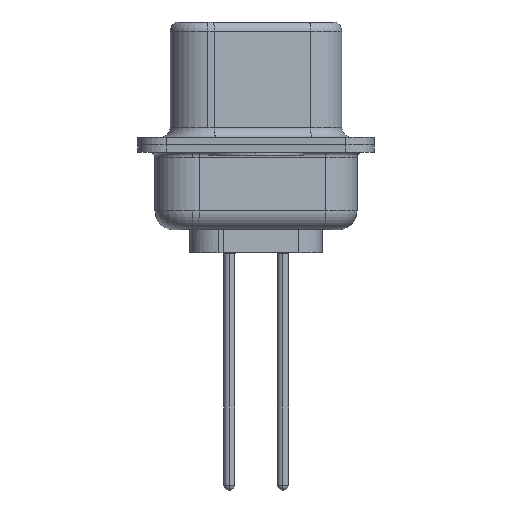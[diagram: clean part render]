
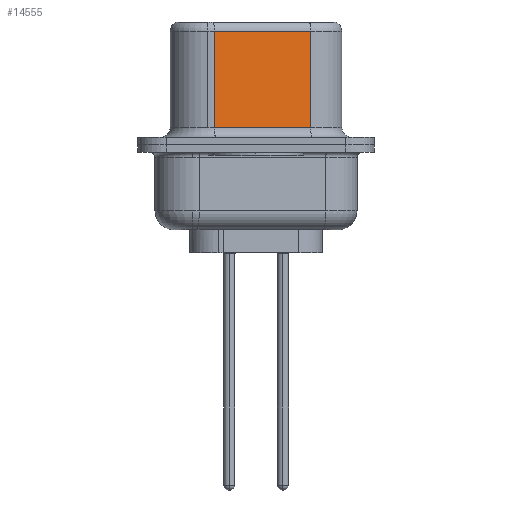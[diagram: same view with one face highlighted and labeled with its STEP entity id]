
A CAD part, left-side view. The second image highlights one B-rep face of the part: STEP entity #14555.
In plain terms, the highlighted planar face has unit normal (-0.985, -0.174, 0).
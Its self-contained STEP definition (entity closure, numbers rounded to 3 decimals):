
#50 = CARTESIAN_POINT ( 'NONE',  ( 4.58, -2.897, 6.02 ) ) ;
#184 = DIRECTION ( 'NONE',  ( 0.174, -0.985, 0. ) ) ;
#519 = AXIS2_PLACEMENT_3D ( 'NONE', #16702, #12219, #586 ) ;
#586 = DIRECTION ( 'NONE',  ( -0.174, 0.985, 0. ) ) ;
#2310 = VECTOR ( 'NONE', #7303, 1000. ) ;
#2492 = CARTESIAN_POINT ( 'NONE',  ( 4.58, -2.897, 0.9 ) ) ;
#3308 = ORIENTED_EDGE ( 'NONE', *, *, #7436, .F. ) ;
#3368 = ORIENTED_EDGE ( 'NONE', *, *, #14794, .T. ) ;
#3819 = VECTOR ( 'NONE', #14747, 1000. ) ;
#4677 = LINE ( 'NONE', #7627, #6140 ) ;
#4984 = PLANE ( 'NONE',  #519 ) ;
#5280 = EDGE_LOOP ( 'NONE', ( #3308, #17584, #11274, #3368 ) ) ;
#5916 = EDGE_CURVE ( 'NONE', #13630, #14020, #14554, .T. ) ;
#6140 = VECTOR ( 'NONE', #13435, 1000. ) ;
#6310 = CARTESIAN_POINT ( 'NONE',  ( 4.58, -2.897, 0.9 ) ) ;
#6326 = VERTEX_POINT ( 'NONE', #14723 ) ;
#6964 = VERTEX_POINT ( 'NONE', #6310 ) ;
#7303 = DIRECTION ( 'NONE',  ( -0.174, 0.985, 0. ) ) ;
#7436 = EDGE_CURVE ( 'NONE', #13630, #6964, #4677, .T. ) ;
#7627 = CARTESIAN_POINT ( 'NONE',  ( 4.58, -2.897, 6.52 ) ) ;
#10887 = FACE_OUTER_BOUND ( 'NONE', #5280, .T. ) ;
#11274 = ORIENTED_EDGE ( 'NONE', *, *, #17040, .T. ) ;
#12219 = DIRECTION ( 'NONE',  ( 0.985, 0.174, 0. ) ) ;
#13435 = DIRECTION ( 'NONE',  ( 0., 0., -1. ) ) ;
#13630 = VERTEX_POINT ( 'NONE', #16355 ) ;
#14020 = VERTEX_POINT ( 'NONE', #15855 ) ;
#14547 = VECTOR ( 'NONE', #184, 1000. ) ;
#14554 = LINE ( 'NONE', #50, #2310 ) ;
#14555 = ADVANCED_FACE ( 'NONE', ( #10887 ), #4984, .F. ) ;
#14657 = LINE ( 'NONE', #17605, #3819 ) ;
#14723 = CARTESIAN_POINT ( 'NONE',  ( 3.68, 2.203, 0.9 ) ) ;
#14747 = DIRECTION ( 'NONE',  ( 0., 0., -1. ) ) ;
#14794 = EDGE_CURVE ( 'NONE', #6326, #6964, #18694, .T. ) ;
#15855 = CARTESIAN_POINT ( 'NONE',  ( 3.68, 2.203, 6.02 ) ) ;
#16355 = CARTESIAN_POINT ( 'NONE',  ( 4.58, -2.897, 6.02 ) ) ;
#16702 = CARTESIAN_POINT ( 'NONE',  ( 4.58, -2.897, 6.52 ) ) ;
#17040 = EDGE_CURVE ( 'NONE', #14020, #6326, #14657, .T. ) ;
#17584 = ORIENTED_EDGE ( 'NONE', *, *, #5916, .T. ) ;
#17605 = CARTESIAN_POINT ( 'NONE',  ( 3.68, 2.203, 6.52 ) ) ;
#18694 = LINE ( 'NONE', #2492, #14547 ) ;
